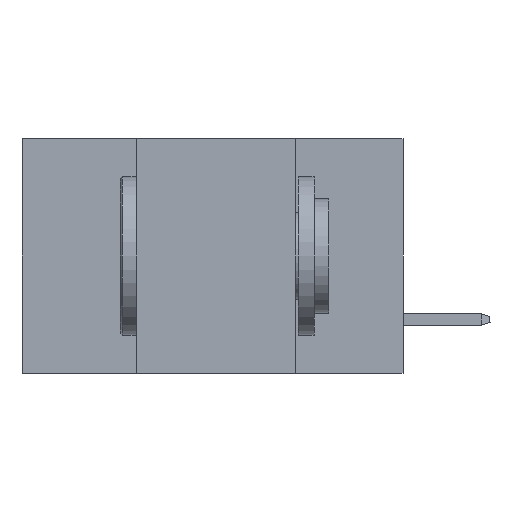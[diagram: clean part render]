
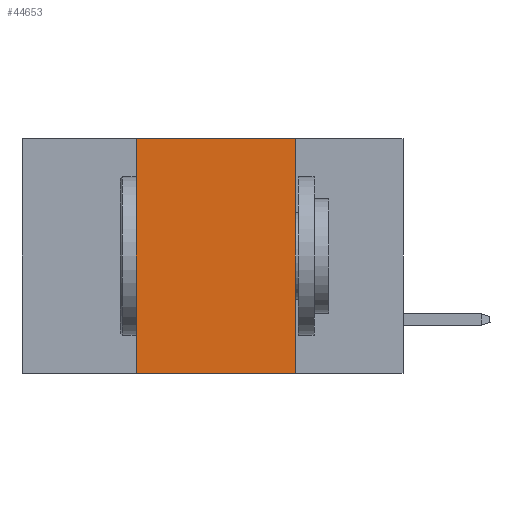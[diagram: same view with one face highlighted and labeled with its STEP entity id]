
A CAD part, left-side view. The second image highlights one B-rep face of the part: STEP entity #44653.
In plain terms, the highlighted planar face has unit normal (-1, 0, 0).
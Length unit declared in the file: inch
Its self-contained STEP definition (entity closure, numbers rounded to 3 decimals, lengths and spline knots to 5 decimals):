
#1240 = VECTOR ( 'NONE', #30600, 39.37008 ) ;
#1800 = VERTEX_POINT ( 'NONE', #1891 ) ;
#1891 = CARTESIAN_POINT ( 'NONE',  ( 0., 0.42, -0.37 ) ) ;
#3263 = EDGE_CURVE ( 'NONE', #11991, #15074, #35252, .T. ) ;
#5253 = DIRECTION ( 'NONE',  ( 0., -1., 0. ) ) ;
#5958 = VECTOR ( 'NONE', #28619, 39.37008 ) ;
#9544 = PLANE ( 'NONE',  #17875 ) ;
#10487 = DIRECTION ( 'NONE',  ( 0., 0., -1. ) ) ;
#11991 = VERTEX_POINT ( 'NONE', #19245 ) ;
#12847 = LINE ( 'NONE', #41415, #33988 ) ;
#14339 = ORIENTED_EDGE ( 'NONE', *, *, #3263, .F. ) ;
#15074 = VERTEX_POINT ( 'NONE', #37442 ) ;
#16909 = DIRECTION ( 'NONE',  ( 1., 0., 0. ) ) ;
#17875 = AXIS2_PLACEMENT_3D ( 'NONE', #39499, #16909, #10487 ) ;
#17985 = EDGE_CURVE ( 'NONE', #1800, #11991, #42132, .T. ) ;
#18011 = CARTESIAN_POINT ( 'NONE',  ( 0., 0.17, -0.37 ) ) ;
#19245 = CARTESIAN_POINT ( 'NONE',  ( 0., 0.42, 0. ) ) ;
#19762 = EDGE_CURVE ( 'NONE', #15074, #30925, #46351, .T. ) ;
#24887 = CARTESIAN_POINT ( 'NONE',  ( 0., 0.6, 0. ) ) ;
#27718 = FACE_OUTER_BOUND ( 'NONE', #28841, .T. ) ;
#28619 = DIRECTION ( 'NONE',  ( 0., 0., -1. ) ) ;
#28841 = EDGE_LOOP ( 'NONE', ( #44474, #14339, #29512, #39168 ) ) ;
#29512 = ORIENTED_EDGE ( 'NONE', *, *, #17985, .F. ) ;
#30401 = VECTOR ( 'NONE', #46223, 39.37008 ) ;
#30600 = DIRECTION ( 'NONE',  ( 0., 0., 1. ) ) ;
#30925 = VERTEX_POINT ( 'NONE', #18011 ) ;
#33988 = VECTOR ( 'NONE', #5253, 39.37008 ) ;
#35252 = LINE ( 'NONE', #24887, #30401 ) ;
#37442 = CARTESIAN_POINT ( 'NONE',  ( 0., 0.17, 0. ) ) ;
#38536 = CARTESIAN_POINT ( 'NONE',  ( 0., 0.42, 0. ) ) ;
#39168 = ORIENTED_EDGE ( 'NONE', *, *, #44419, .T. ) ;
#39499 = CARTESIAN_POINT ( 'NONE',  ( 0., 0.6, 0. ) ) ;
#41415 = CARTESIAN_POINT ( 'NONE',  ( 0., 0.6, -0.37 ) ) ;
#42132 = LINE ( 'NONE', #38536, #1240 ) ;
#44419 = EDGE_CURVE ( 'NONE', #1800, #30925, #12847, .T. ) ;
#44474 = ORIENTED_EDGE ( 'NONE', *, *, #19762, .F. ) ;
#44653 = ADVANCED_FACE ( 'NONE', ( #27718 ), #9544, .F. ) ;
#46223 = DIRECTION ( 'NONE',  ( 0., -1., 0. ) ) ;
#46351 = LINE ( 'NONE', #46836, #5958 ) ;
#46836 = CARTESIAN_POINT ( 'NONE',  ( 0., 0.17, 0. ) ) ;
